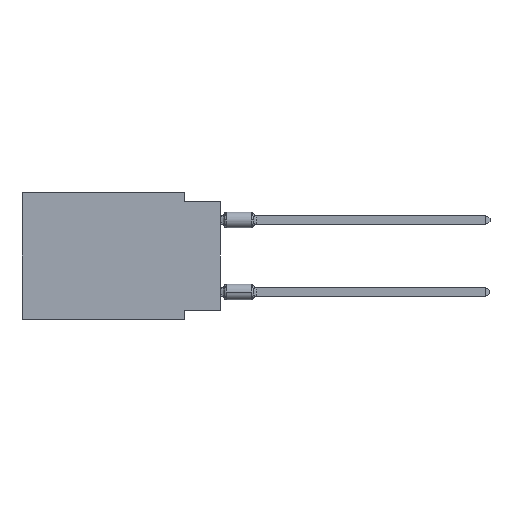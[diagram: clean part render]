
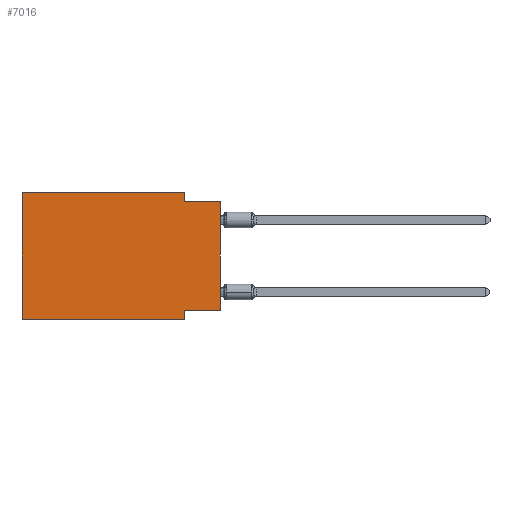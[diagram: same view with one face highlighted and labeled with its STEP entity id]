
A CAD part, left-side view. The second image highlights one B-rep face of the part: STEP entity #7016.
In plain terms, the highlighted planar face has unit normal (-1, 0, 0).
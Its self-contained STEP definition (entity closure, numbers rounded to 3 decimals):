
#367 = CARTESIAN_POINT ( 'NONE',  ( 0., 13.97, -8.89 ) ) ;
#740 = EDGE_CURVE ( 'NONE', #4802, #7040, #8925, .T. ) ;
#1687 = VERTEX_POINT ( 'NONE', #8106 ) ;
#2010 = ORIENTED_EDGE ( 'NONE', *, *, #9529, .F. ) ;
#2016 = ORIENTED_EDGE ( 'NONE', *, *, #740, .F. ) ;
#2119 = DIRECTION ( 'NONE',  ( 0., -1., 0. ) ) ;
#2198 = VERTEX_POINT ( 'NONE', #12439 ) ;
#2514 = CARTESIAN_POINT ( 'NONE',  ( 0., 13.97, 0. ) ) ;
#2607 = DIRECTION ( 'NONE',  ( 0., -1., 0. ) ) ;
#2725 = CARTESIAN_POINT ( 'NONE',  ( 0., 2.54, -0.635 ) ) ;
#2825 = VECTOR ( 'NONE', #7562, 1000. ) ;
#2863 = LINE ( 'NONE', #9193, #4670 ) ;
#3131 = VECTOR ( 'NONE', #2119, 1000. ) ;
#3348 = DIRECTION ( 'NONE',  ( 0., 1., 0. ) ) ;
#3519 = ORIENTED_EDGE ( 'NONE', *, *, #6451, .F. ) ;
#4670 = VECTOR ( 'NONE', #13390, 1000. ) ;
#4745 = EDGE_CURVE ( 'NONE', #6775, #1687, #5355, .T. ) ;
#4802 = VERTEX_POINT ( 'NONE', #7673 ) ;
#5128 = DIRECTION ( 'NONE',  ( 1., 0., 0. ) ) ;
#5355 = LINE ( 'NONE', #12912, #6079 ) ;
#5367 = DIRECTION ( 'NONE',  ( 0., 0., -1. ) ) ;
#5564 = EDGE_LOOP ( 'NONE', ( #7578, #3519, #6785, #2016, #2010, #10381, #13127, #11849 ) ) ;
#5921 = CARTESIAN_POINT ( 'NONE',  ( 0., 2.54, -8.89 ) ) ;
#6079 = VECTOR ( 'NONE', #3348, 1000. ) ;
#6205 = VERTEX_POINT ( 'NONE', #10346 ) ;
#6407 = CARTESIAN_POINT ( 'NONE',  ( 0., 13.97, 0. ) ) ;
#6446 = CARTESIAN_POINT ( 'NONE',  ( 0., 0., -8.255 ) ) ;
#6451 = EDGE_CURVE ( 'NONE', #10964, #6205, #6934, .T. ) ;
#6711 = DIRECTION ( 'NONE',  ( 0., 0., 1. ) ) ;
#6775 = VERTEX_POINT ( 'NONE', #6446 ) ;
#6785 = ORIENTED_EDGE ( 'NONE', *, *, #10967, .F. ) ;
#6924 = CARTESIAN_POINT ( 'NONE',  ( 0., 13.97, 0. ) ) ;
#6934 = LINE ( 'NONE', #12999, #7221 ) ;
#7016 = ADVANCED_FACE ( 'NONE', ( #10366 ), #11654, .F. ) ;
#7025 = VECTOR ( 'NONE', #8510, 1000. ) ;
#7040 = VERTEX_POINT ( 'NONE', #7577 ) ;
#7213 = LINE ( 'NONE', #11621, #7025 ) ;
#7221 = VECTOR ( 'NONE', #2607, 1000. ) ;
#7553 = EDGE_CURVE ( 'NONE', #2198, #8837, #9702, .T. ) ;
#7562 = DIRECTION ( 'NONE',  ( 0., -1., 0. ) ) ;
#7577 = CARTESIAN_POINT ( 'NONE',  ( 0., 2.54, 0. ) ) ;
#7578 = ORIENTED_EDGE ( 'NONE', *, *, #9078, .T. ) ;
#7673 = CARTESIAN_POINT ( 'NONE',  ( 0., 13.97, 0. ) ) ;
#8106 = CARTESIAN_POINT ( 'NONE',  ( 0., 2.54, -8.255 ) ) ;
#8147 = VECTOR ( 'NONE', #6711, 1000. ) ;
#8510 = DIRECTION ( 'NONE',  ( 0., 0., 1. ) ) ;
#8613 = DIRECTION ( 'NONE',  ( 0., 0., -1. ) ) ;
#8703 = LINE ( 'NONE', #2514, #8147 ) ;
#8837 = VERTEX_POINT ( 'NONE', #5921 ) ;
#8925 = LINE ( 'NONE', #6924, #3131 ) ;
#9078 = EDGE_CURVE ( 'NONE', #6775, #6205, #7213, .T. ) ;
#9193 = CARTESIAN_POINT ( 'NONE',  ( 0., 2.54, 0. ) ) ;
#9529 = EDGE_CURVE ( 'NONE', #2198, #4802, #8703, .T. ) ;
#9702 = LINE ( 'NONE', #367, #2825 ) ;
#10346 = CARTESIAN_POINT ( 'NONE',  ( 0., 0., -0.635 ) ) ;
#10366 = FACE_OUTER_BOUND ( 'NONE', #5564, .T. ) ;
#10381 = ORIENTED_EDGE ( 'NONE', *, *, #7553, .T. ) ;
#10667 = LINE ( 'NONE', #12715, #13469 ) ;
#10964 = VERTEX_POINT ( 'NONE', #2725 ) ;
#10967 = EDGE_CURVE ( 'NONE', #7040, #10964, #2863, .T. ) ;
#11621 = CARTESIAN_POINT ( 'NONE',  ( 0., 0., 0. ) ) ;
#11654 = PLANE ( 'NONE',  #11858 ) ;
#11849 = ORIENTED_EDGE ( 'NONE', *, *, #4745, .F. ) ;
#11858 = AXIS2_PLACEMENT_3D ( 'NONE', #6407, #5128, #8613 ) ;
#11907 = EDGE_CURVE ( 'NONE', #1687, #8837, #10667, .T. ) ;
#12439 = CARTESIAN_POINT ( 'NONE',  ( 0., 13.97, -8.89 ) ) ;
#12715 = CARTESIAN_POINT ( 'NONE',  ( 0., 2.54, -8.89 ) ) ;
#12912 = CARTESIAN_POINT ( 'NONE',  ( 0., 0., -8.255 ) ) ;
#12999 = CARTESIAN_POINT ( 'NONE',  ( 0., 0., -0.635 ) ) ;
#13127 = ORIENTED_EDGE ( 'NONE', *, *, #11907, .F. ) ;
#13390 = DIRECTION ( 'NONE',  ( 0., 0., -1. ) ) ;
#13469 = VECTOR ( 'NONE', #5367, 1000. ) ;
